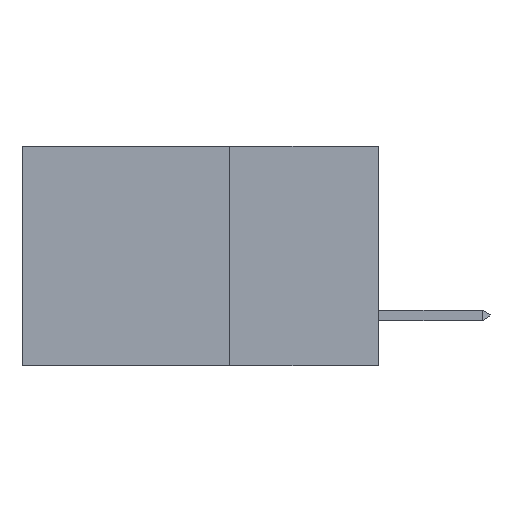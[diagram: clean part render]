
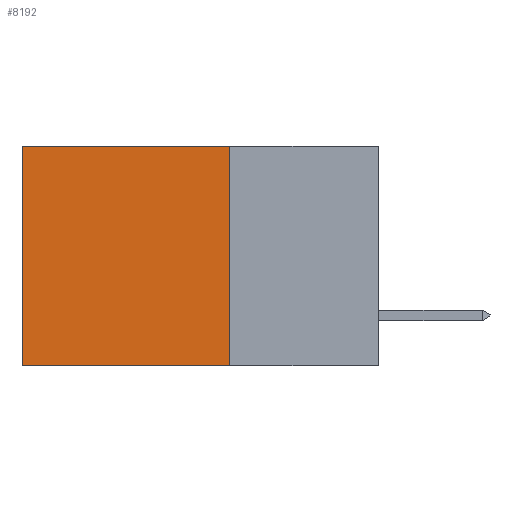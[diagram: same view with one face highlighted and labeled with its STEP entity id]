
A CAD part, left-side view. The second image highlights one B-rep face of the part: STEP entity #8192.
In plain terms, the highlighted planar face has unit normal (-1, 0, 0).
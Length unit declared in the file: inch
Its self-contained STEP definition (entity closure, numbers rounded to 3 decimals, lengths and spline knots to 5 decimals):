
#462 = DIRECTION ( 'NONE',  ( 0., 0., -1. ) ) ;
#477 = CARTESIAN_POINT ( 'NONE',  ( 0.298, 0.25, -0.37 ) ) ;
#497 = CARTESIAN_POINT ( 'NONE',  ( 0.298, 0.6, 0. ) ) ;
#768 = ORIENTED_EDGE ( 'NONE', *, *, #8096, .T. ) ;
#1601 = LINE ( 'NONE', #477, #6340 ) ;
#1624 = VECTOR ( 'NONE', #10776, 39.37008 ) ;
#3362 = CARTESIAN_POINT ( 'NONE',  ( 0.298, 0.25, 0. ) ) ;
#3435 = EDGE_CURVE ( 'NONE', #10514, #7915, #8015, .T. ) ;
#3698 = CARTESIAN_POINT ( 'NONE',  ( 0.298, 0.25, 0. ) ) ;
#3788 = LINE ( 'NONE', #497, #9997 ) ;
#3838 = LINE ( 'NONE', #6923, #1624 ) ;
#4433 = FACE_OUTER_BOUND ( 'NONE', #7907, .T. ) ;
#4774 = CARTESIAN_POINT ( 'NONE',  ( 0.298, 0.6, -0.37 ) ) ;
#5148 = DIRECTION ( 'NONE',  ( 0., 0., -1. ) ) ;
#5539 = EDGE_CURVE ( 'NONE', #7915, #11687, #1601, .T. ) ;
#6112 = ORIENTED_EDGE ( 'NONE', *, *, #6346, .T. ) ;
#6161 = VERTEX_POINT ( 'NONE', #11746 ) ;
#6169 = PLANE ( 'NONE',  #11128 ) ;
#6340 = VECTOR ( 'NONE', #8988, 39.37008 ) ;
#6346 = EDGE_CURVE ( 'NONE', #6161, #11687, #3788, .T. ) ;
#6681 = DIRECTION ( 'NONE',  ( 0., 0., -1. ) ) ;
#6698 = VECTOR ( 'NONE', #6681, 39.37008 ) ;
#6923 = CARTESIAN_POINT ( 'NONE',  ( 0.298, 0.25, 0. ) ) ;
#7162 = CARTESIAN_POINT ( 'NONE',  ( 0.298, 0.25, 0. ) ) ;
#7907 = EDGE_LOOP ( 'NONE', ( #6112, #8482, #10642, #768 ) ) ;
#7915 = VERTEX_POINT ( 'NONE', #9370 ) ;
#8015 = LINE ( 'NONE', #3698, #6698 ) ;
#8096 = EDGE_CURVE ( 'NONE', #10514, #6161, #3838, .T. ) ;
#8192 = ADVANCED_FACE ( 'NONE', ( #4433 ), #6169, .F. ) ;
#8482 = ORIENTED_EDGE ( 'NONE', *, *, #5539, .F. ) ;
#8889 = DIRECTION ( 'NONE',  ( 1., 0., 0. ) ) ;
#8988 = DIRECTION ( 'NONE',  ( 0., 1., 0. ) ) ;
#9370 = CARTESIAN_POINT ( 'NONE',  ( 0.298, 0.25, -0.37 ) ) ;
#9997 = VECTOR ( 'NONE', #462, 39.37008 ) ;
#10514 = VERTEX_POINT ( 'NONE', #7162 ) ;
#10642 = ORIENTED_EDGE ( 'NONE', *, *, #3435, .F. ) ;
#10776 = DIRECTION ( 'NONE',  ( 0., 1., 0. ) ) ;
#11128 = AXIS2_PLACEMENT_3D ( 'NONE', #3362, #8889, #5148 ) ;
#11687 = VERTEX_POINT ( 'NONE', #4774 ) ;
#11746 = CARTESIAN_POINT ( 'NONE',  ( 0.298, 0.6, 0. ) ) ;
